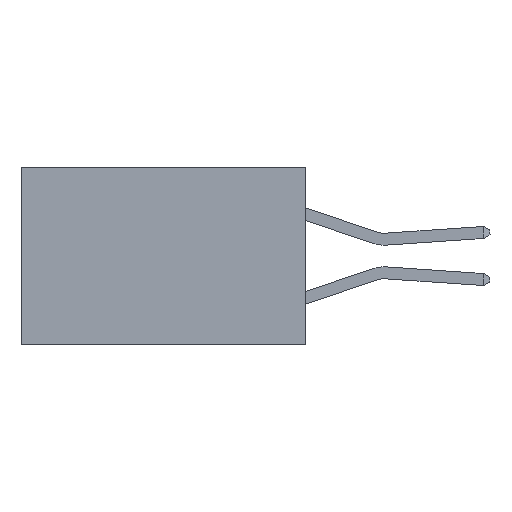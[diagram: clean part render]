
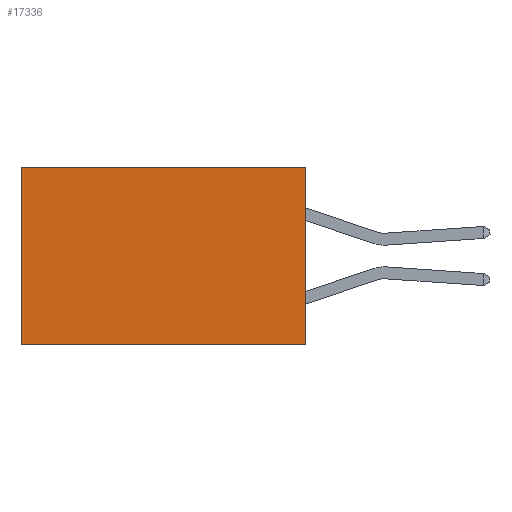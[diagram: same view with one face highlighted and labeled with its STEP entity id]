
A CAD part, left-side view. The second image highlights one B-rep face of the part: STEP entity #17336.
In plain terms, the highlighted planar face has unit normal (-1, 0, 0).
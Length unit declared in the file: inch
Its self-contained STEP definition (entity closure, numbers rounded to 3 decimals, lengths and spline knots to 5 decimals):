
#194 = EDGE_CURVE ( 'NONE', #7353, #19880, #26143, .T. ) ;
#701 = PLANE ( 'NONE',  #16062 ) ;
#1277 = DIRECTION ( 'NONE',  ( 0., 1., 0. ) ) ;
#2048 = CARTESIAN_POINT ( 'NONE',  ( 0.277, 0.59, 0. ) ) ;
#3489 = ORIENTED_EDGE ( 'NONE', *, *, #20632, .T. ) ;
#4516 = LINE ( 'NONE', #17914, #29196 ) ;
#5485 = DIRECTION ( 'NONE',  ( 1., 0., 0. ) ) ;
#5920 = DIRECTION ( 'NONE',  ( 0., 0., -1. ) ) ;
#6240 = VECTOR ( 'NONE', #29592, 39.37008 ) ;
#6563 = EDGE_LOOP ( 'NONE', ( #3489, #18998, #22107, #16354 ) ) ;
#6579 = VERTEX_POINT ( 'NONE', #11907 ) ;
#7125 = DIRECTION ( 'NONE',  ( 0., 1., 0. ) ) ;
#7353 = VERTEX_POINT ( 'NONE', #25481 ) ;
#9227 = CARTESIAN_POINT ( 'NONE',  ( 0.277, 0., -0.37 ) ) ;
#10750 = VECTOR ( 'NONE', #7125, 39.37008 ) ;
#11650 = EDGE_CURVE ( 'NONE', #19880, #6579, #14792, .T. ) ;
#11907 = CARTESIAN_POINT ( 'NONE',  ( 0.277, 0.59, -0.37 ) ) ;
#14792 = LINE ( 'NONE', #22888, #26785 ) ;
#16062 = AXIS2_PLACEMENT_3D ( 'NONE', #19879, #5485, #22300 ) ;
#16354 = ORIENTED_EDGE ( 'NONE', *, *, #28353, .T. ) ;
#17336 = ADVANCED_FACE ( 'NONE', ( #30386 ), #701, .F. ) ;
#17914 = CARTESIAN_POINT ( 'NONE',  ( 0.277, 0.59, -0.37 ) ) ;
#18998 = ORIENTED_EDGE ( 'NONE', *, *, #11650, .F. ) ;
#19114 = CARTESIAN_POINT ( 'NONE',  ( 0.277, 0., 0. ) ) ;
#19879 = CARTESIAN_POINT ( 'NONE',  ( 0.277, 0., -0.37 ) ) ;
#19880 = VERTEX_POINT ( 'NONE', #21963 ) ;
#20632 = EDGE_CURVE ( 'NONE', #30267, #6579, #4516, .T. ) ;
#21963 = CARTESIAN_POINT ( 'NONE',  ( 0.277, 0., -0.37 ) ) ;
#22107 = ORIENTED_EDGE ( 'NONE', *, *, #194, .F. ) ;
#22300 = DIRECTION ( 'NONE',  ( 0., 0., -1. ) ) ;
#22888 = CARTESIAN_POINT ( 'NONE',  ( 0.277, 0., -0.37 ) ) ;
#23583 = LINE ( 'NONE', #19114, #10750 ) ;
#25481 = CARTESIAN_POINT ( 'NONE',  ( 0.277, 0., 0. ) ) ;
#26143 = LINE ( 'NONE', #9227, #6240 ) ;
#26785 = VECTOR ( 'NONE', #1277, 39.37008 ) ;
#28353 = EDGE_CURVE ( 'NONE', #7353, #30267, #23583, .T. ) ;
#29196 = VECTOR ( 'NONE', #5920, 39.37008 ) ;
#29592 = DIRECTION ( 'NONE',  ( 0., 0., -1. ) ) ;
#30267 = VERTEX_POINT ( 'NONE', #2048 ) ;
#30386 = FACE_OUTER_BOUND ( 'NONE', #6563, .T. ) ;
